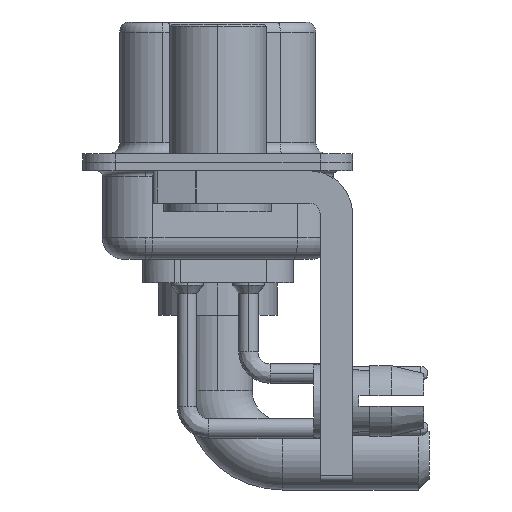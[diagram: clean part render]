
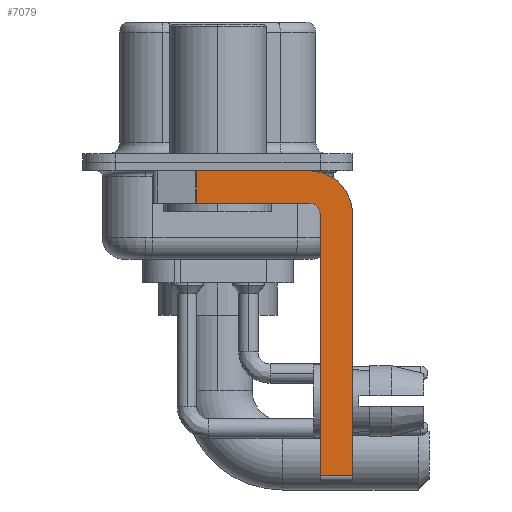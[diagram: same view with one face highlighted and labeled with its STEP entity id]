
A CAD part, left-side view. The second image highlights one B-rep face of the part: STEP entity #7079.
In plain terms, the highlighted planar face has unit normal (-1, 0, 0).
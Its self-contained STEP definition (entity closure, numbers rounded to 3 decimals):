
#1156 = DIRECTION ( 'NONE',  ( -1., 0., 0. ) ) ;
#1764 = ORIENTED_EDGE ( 'NONE', *, *, #23170, .F. ) ;
#2314 = VERTEX_POINT ( 'NONE', #29112 ) ;
#3803 = LINE ( 'NONE', #4781, #12319 ) ;
#4240 = DIRECTION ( 'NONE',  ( 0., 1., 0. ) ) ;
#4781 = CARTESIAN_POINT ( 'NONE',  ( -2.9, -4.75, -14.8 ) ) ;
#5215 = DIRECTION ( 'NONE',  ( 1., 0., 0. ) ) ;
#5481 = ORIENTED_EDGE ( 'NONE', *, *, #19752, .T. ) ;
#6136 = DIRECTION ( 'NONE',  ( 0., 0., -1. ) ) ;
#7079 = ADVANCED_FACE ( 'NONE', ( #10168 ), #10606, .F. ) ;
#8466 = AXIS2_PLACEMENT_3D ( 'NONE', #23081, #5215, #9834 ) ;
#8724 = DIRECTION ( 'NONE',  ( 0., -1., 0. ) ) ;
#8967 = VECTOR ( 'NONE', #12005, 1000. ) ;
#9158 = CARTESIAN_POINT ( 'NONE',  ( -2.9, 3., -0.4 ) ) ;
#9470 = LINE ( 'NONE', #18545, #8967 ) ;
#9784 = CIRCLE ( 'NONE', #13588, 0.5 ) ;
#9834 = DIRECTION ( 'NONE',  ( 0., 0., -1. ) ) ;
#10143 = VERTEX_POINT ( 'NONE', #17420 ) ;
#10168 = FACE_OUTER_BOUND ( 'NONE', #21738, .T. ) ;
#10395 = ORIENTED_EDGE ( 'NONE', *, *, #20592, .T. ) ;
#10562 = ORIENTED_EDGE ( 'NONE', *, *, #18874, .F. ) ;
#10606 = PLANE ( 'NONE',  #29150 ) ;
#10943 = LINE ( 'NONE', #20174, #28235 ) ;
#11592 = CARTESIAN_POINT ( 'NONE',  ( -2.9, 0.978, -1.9 ) ) ;
#12005 = DIRECTION ( 'NONE',  ( 0., 0., -1. ) ) ;
#12087 = VECTOR ( 'NONE', #22907, 1000. ) ;
#12319 = VECTOR ( 'NONE', #15275, 1000. ) ;
#13588 = AXIS2_PLACEMENT_3D ( 'NONE', #21544, #1156, #18862 ) ;
#13611 = ORIENTED_EDGE ( 'NONE', *, *, #19225, .F. ) ;
#13735 = CARTESIAN_POINT ( 'NONE',  ( -2.9, -4.25, -0.4 ) ) ;
#14055 = VERTEX_POINT ( 'NONE', #28543 ) ;
#15073 = VERTEX_POINT ( 'NONE', #24445 ) ;
#15275 = DIRECTION ( 'NONE',  ( 0., 0., 1. ) ) ;
#15430 = LINE ( 'NONE', #9158, #26137 ) ;
#15888 = VERTEX_POINT ( 'NONE', #16513 ) ;
#16513 = CARTESIAN_POINT ( 'NONE',  ( -2.9, -6.25, -2.4 ) ) ;
#16587 = ORIENTED_EDGE ( 'NONE', *, *, #26841, .F. ) ;
#17420 = CARTESIAN_POINT ( 'NONE',  ( -2.9, -4.25, -1.9 ) ) ;
#17457 = CARTESIAN_POINT ( 'NONE',  ( -2.9, -4.25, -2.4 ) ) ;
#17975 = CIRCLE ( 'NONE', #8466, 2. ) ;
#18030 = EDGE_CURVE ( 'NONE', #27455, #15888, #17975, .T. ) ;
#18545 = CARTESIAN_POINT ( 'NONE',  ( -2.9, -6.25, -2.4 ) ) ;
#18862 = DIRECTION ( 'NONE',  ( 0., 0., 1. ) ) ;
#18874 = EDGE_CURVE ( 'NONE', #15888, #14055, #9470, .T. ) ;
#19225 = EDGE_CURVE ( 'NONE', #15073, #20463, #3803, .T. ) ;
#19752 = EDGE_CURVE ( 'NONE', #20635, #2314, #23049, .T. ) ;
#20174 = CARTESIAN_POINT ( 'NONE',  ( -2.9, -4.25, -1.9 ) ) ;
#20411 = EDGE_CURVE ( 'NONE', #10143, #2314, #10943, .T. ) ;
#20463 = VERTEX_POINT ( 'NONE', #22989 ) ;
#20592 = EDGE_CURVE ( 'NONE', #15073, #14055, #23865, .T. ) ;
#20635 = VERTEX_POINT ( 'NONE', #25813 ) ;
#21544 = CARTESIAN_POINT ( 'NONE',  ( -2.9, -4.25, -2.4 ) ) ;
#21738 = EDGE_LOOP ( 'NONE', ( #16587, #5481, #27397, #1764, #13611, #10395, #10562, #29245 ) ) ;
#22907 = DIRECTION ( 'NONE',  ( 0., 0., -1. ) ) ;
#22989 = CARTESIAN_POINT ( 'NONE',  ( -2.9, -4.75, -2.4 ) ) ;
#23049 = LINE ( 'NONE', #11592, #12087 ) ;
#23081 = CARTESIAN_POINT ( 'NONE',  ( -2.9, -4.25, -2.4 ) ) ;
#23170 = EDGE_CURVE ( 'NONE', #20463, #10143, #9784, .T. ) ;
#23865 = LINE ( 'NONE', #28774, #27330 ) ;
#24445 = CARTESIAN_POINT ( 'NONE',  ( -2.9, -4.75, -14.55 ) ) ;
#25813 = CARTESIAN_POINT ( 'NONE',  ( -2.9, 0.978, -0.4 ) ) ;
#26137 = VECTOR ( 'NONE', #8724, 1000. ) ;
#26525 = DIRECTION ( 'NONE',  ( 1., 0., 0. ) ) ;
#26841 = EDGE_CURVE ( 'NONE', #20635, #27455, #15430, .T. ) ;
#27330 = VECTOR ( 'NONE', #28181, 1000. ) ;
#27397 = ORIENTED_EDGE ( 'NONE', *, *, #20411, .F. ) ;
#27455 = VERTEX_POINT ( 'NONE', #13735 ) ;
#28181 = DIRECTION ( 'NONE',  ( 0., -1., 0. ) ) ;
#28235 = VECTOR ( 'NONE', #4240, 1000. ) ;
#28543 = CARTESIAN_POINT ( 'NONE',  ( -2.9, -6.25, -14.55 ) ) ;
#28774 = CARTESIAN_POINT ( 'NONE',  ( -2.9, -4.25, -14.55 ) ) ;
#29112 = CARTESIAN_POINT ( 'NONE',  ( -2.9, 0.978, -1.9 ) ) ;
#29150 = AXIS2_PLACEMENT_3D ( 'NONE', #17457, #26525, #6136 ) ;
#29245 = ORIENTED_EDGE ( 'NONE', *, *, #18030, .F. ) ;
